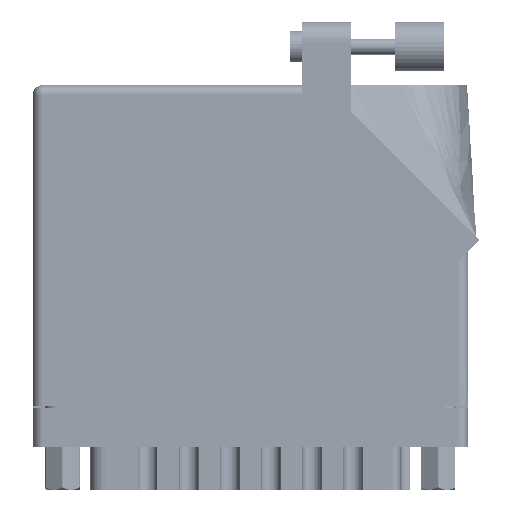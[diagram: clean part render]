
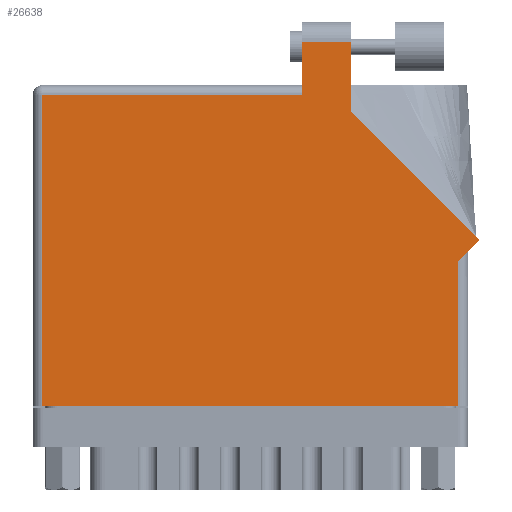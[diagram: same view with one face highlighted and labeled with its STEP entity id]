
A CAD part, front view. The second image highlights one B-rep face of the part: STEP entity #26638.
In plain terms, the highlighted face is planar.
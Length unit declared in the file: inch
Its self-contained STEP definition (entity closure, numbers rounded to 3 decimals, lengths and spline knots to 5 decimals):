
#1036 = DIRECTION ( 'NONE',  ( -0.707, 0.707, 0. ) ) ;
#2984 = CARTESIAN_POINT ( 'NONE',  ( 0.062, 0., 0. ) ) ;
#3780 = EDGE_CURVE ( 'NONE', #6038, #41182, #72877, .T. ) ;
#4057 = DIRECTION ( 'NONE',  ( 0., -1., 0. ) ) ;
#6038 = VERTEX_POINT ( 'NONE', #48321 ) ;
#7956 = DIRECTION ( 'NONE',  ( -1., 0., 0. ) ) ;
#9847 = ORIENTED_EDGE ( 'NONE', *, *, #3780, .T. ) ;
#10489 = LINE ( 'NONE', #14371, #77015 ) ;
#11024 = LINE ( 'NONE', #53865, #63456 ) ;
#12537 = LINE ( 'NONE', #29485, #70073 ) ;
#12552 = EDGE_CURVE ( 'NONE', #54074, #57438, #105897, .T. ) ;
#12867 = LINE ( 'NONE', #51588, #84539 ) ;
#14371 = CARTESIAN_POINT ( 'NONE',  ( 2.82571, 1.05071, 0. ) ) ;
#18445 = ORIENTED_EDGE ( 'NONE', *, *, #54404, .T. ) ;
#18890 = FACE_OUTER_BOUND ( 'NONE', #23339, .T. ) ;
#19541 = ORIENTED_EDGE ( 'NONE', *, *, #35298, .T. ) ;
#20434 = ORIENTED_EDGE ( 'NONE', *, *, #92978, .T. ) ;
#20581 = LINE ( 'NONE', #102301, #58978 ) ;
#22406 = CARTESIAN_POINT ( 'NONE',  ( 0., 0., 0. ) ) ;
#22786 = ORIENTED_EDGE ( 'NONE', *, *, #12552, .T. ) ;
#23339 = EDGE_LOOP ( 'NONE', ( #22786, #68693, #65779, #37931, #18445, #9847, #20434, #19541, #60128 ) ) ;
#23868 = VECTOR ( 'NONE', #29573, 39.37008 ) ;
#24706 = VERTEX_POINT ( 'NONE', #52771 ) ;
#25284 = VERTEX_POINT ( 'NONE', #52329 ) ;
#25771 = VECTOR ( 'NONE', #68081, 39.37008 ) ;
#26140 = AXIS2_PLACEMENT_3D ( 'NONE', #49038, #76314, #27633 ) ;
#26176 = EDGE_CURVE ( 'NONE', #86196, #72549, #99797, .T. ) ;
#26384 = EDGE_CURVE ( 'NONE', #57438, #86196, #12537, .T. ) ;
#26638 = ADVANCED_FACE ( 'NONE', ( #18890 ), #26908, .F. ) ;
#26908 = PLANE ( 'NONE',  #26140 ) ;
#27633 = DIRECTION ( 'NONE',  ( -1., 0., 0. ) ) ;
#27974 = DIRECTION ( 'NONE',  ( 0.707, 0.707, 0. ) ) ;
#29485 = CARTESIAN_POINT ( 'NONE',  ( 1.705, 2.305, 0. ) ) ;
#29573 = DIRECTION ( 'NONE',  ( 0., 1., 0. ) ) ;
#35298 = EDGE_CURVE ( 'NONE', #25284, #72328, #12867, .T. ) ;
#37931 = ORIENTED_EDGE ( 'NONE', *, *, #84709, .T. ) ;
#38826 = DIRECTION ( 'NONE',  ( 1., 0., 0. ) ) ;
#40068 = CARTESIAN_POINT ( 'NONE',  ( 1.705, 1.968, 0. ) ) ;
#41182 = VERTEX_POINT ( 'NONE', #78386 ) ;
#48321 = CARTESIAN_POINT ( 'NONE',  ( 0.062, 0., 0. ) ) ;
#49038 = CARTESIAN_POINT ( 'NONE',  ( 0., 2.03, 0. ) ) ;
#51588 = CARTESIAN_POINT ( 'NONE',  ( 2.755, 0.98, 0. ) ) ;
#52107 = DIRECTION ( 'NONE',  ( -1., 0., 0. ) ) ;
#52329 = CARTESIAN_POINT ( 'NONE',  ( 2.693, 0.918, 0. ) ) ;
#52771 = CARTESIAN_POINT ( 'NONE',  ( 0.062, 1.968, 0. ) ) ;
#53865 = CARTESIAN_POINT ( 'NONE',  ( 2.693, 0.98, 0. ) ) ;
#54074 = VERTEX_POINT ( 'NONE', #78935 ) ;
#54404 = EDGE_CURVE ( 'NONE', #24706, #6038, #70498, .T. ) ;
#55139 = CARTESIAN_POINT ( 'NONE',  ( 2.82571, 1.05071, 0. ) ) ;
#57438 = VERTEX_POINT ( 'NONE', #104040 ) ;
#58978 = VECTOR ( 'NONE', #52107, 39.37008 ) ;
#60128 = ORIENTED_EDGE ( 'NONE', *, *, #67500, .T. ) ;
#63456 = VECTOR ( 'NONE', #78231, 39.37008 ) ;
#65779 = ORIENTED_EDGE ( 'NONE', *, *, #26176, .T. ) ;
#67500 = EDGE_CURVE ( 'NONE', #72328, #54074, #10489, .T. ) ;
#68081 = DIRECTION ( 'NONE',  ( 0., -1., 0. ) ) ;
#68693 = ORIENTED_EDGE ( 'NONE', *, *, #26384, .T. ) ;
#69609 = CARTESIAN_POINT ( 'NONE',  ( 2.012, 1.86442, 0. ) ) ;
#70073 = VECTOR ( 'NONE', #7956, 39.37008 ) ;
#70498 = LINE ( 'NONE', #2984, #25771 ) ;
#72328 = VERTEX_POINT ( 'NONE', #55139 ) ;
#72549 = VERTEX_POINT ( 'NONE', #40068 ) ;
#72877 = LINE ( 'NONE', #22406, #79289 ) ;
#76055 = CARTESIAN_POINT ( 'NONE',  ( 1.705, 2.03, 0. ) ) ;
#76314 = DIRECTION ( 'NONE',  ( 0., 0., -1. ) ) ;
#77015 = VECTOR ( 'NONE', #1036, 39.37008 ) ;
#78231 = DIRECTION ( 'NONE',  ( 0., 1., 0. ) ) ;
#78386 = CARTESIAN_POINT ( 'NONE',  ( 2.693, 0., 0. ) ) ;
#78935 = CARTESIAN_POINT ( 'NONE',  ( 2.012, 1.86442, 0. ) ) ;
#79289 = VECTOR ( 'NONE', #38826, 39.37008 ) ;
#84539 = VECTOR ( 'NONE', #27974, 39.37008 ) ;
#84709 = EDGE_CURVE ( 'NONE', #72549, #24706, #20581, .T. ) ;
#86196 = VERTEX_POINT ( 'NONE', #87257 ) ;
#87257 = CARTESIAN_POINT ( 'NONE',  ( 1.705, 2.305, 0. ) ) ;
#92978 = EDGE_CURVE ( 'NONE', #41182, #25284, #11024, .T. ) ;
#94613 = VECTOR ( 'NONE', #4057, 39.37008 ) ;
#99797 = LINE ( 'NONE', #76055, #94613 ) ;
#102301 = CARTESIAN_POINT ( 'NONE',  ( 0., 1.968, 0. ) ) ;
#104040 = CARTESIAN_POINT ( 'NONE',  ( 2.012, 2.305, 0. ) ) ;
#105897 = LINE ( 'NONE', #69609, #23868 ) ;
